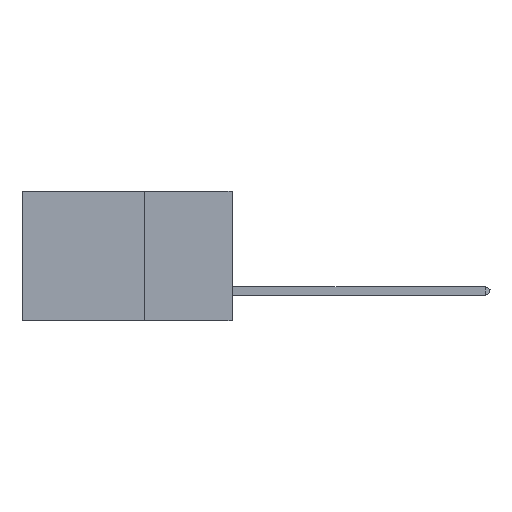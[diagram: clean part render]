
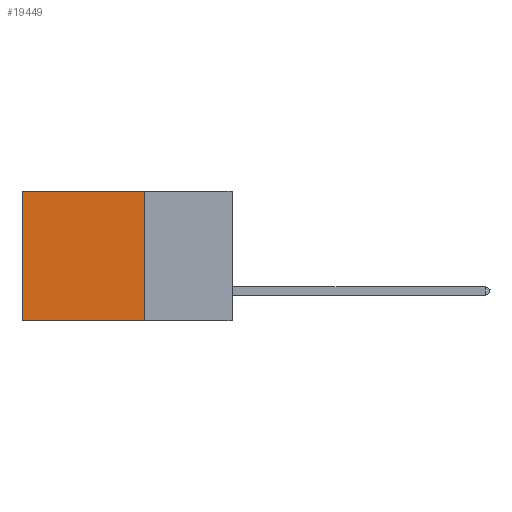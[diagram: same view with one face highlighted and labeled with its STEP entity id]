
A CAD part, left-side view. The second image highlights one B-rep face of the part: STEP entity #19449.
In plain terms, the highlighted planar face has unit normal (-1, 0, 0).
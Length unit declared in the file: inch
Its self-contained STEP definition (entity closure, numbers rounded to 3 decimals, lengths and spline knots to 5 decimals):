
#195 = ORIENTED_EDGE ( 'NONE', *, *, #9380, .F. ) ;
#300 = EDGE_CURVE ( 'NONE', #11918, #4703, #20986, .T. ) ;
#699 = VERTEX_POINT ( 'NONE', #17692 ) ;
#1132 = DIRECTION ( 'NONE',  ( 0., 1., 0. ) ) ;
#1620 = AXIS2_PLACEMENT_3D ( 'NONE', #14199, #4064, #3139 ) ;
#2274 = VERTEX_POINT ( 'NONE', #18508 ) ;
#2371 = EDGE_CURVE ( 'NONE', #4703, #2274, #4594, .T. ) ;
#3139 = DIRECTION ( 'NONE',  ( 0., 0., -1. ) ) ;
#3209 = CARTESIAN_POINT ( 'NONE',  ( 0.2875, 0.6, 0. ) ) ;
#3316 = CARTESIAN_POINT ( 'NONE',  ( 0.2875, 0.25, 0. ) ) ;
#3776 = CARTESIAN_POINT ( 'NONE',  ( 0.2875, 0.25, -0.37 ) ) ;
#4064 = DIRECTION ( 'NONE',  ( 1., 0., 0. ) ) ;
#4594 = LINE ( 'NONE', #5502, #14219 ) ;
#4656 = LINE ( 'NONE', #3316, #12672 ) ;
#4703 = VERTEX_POINT ( 'NONE', #3209 ) ;
#5502 = CARTESIAN_POINT ( 'NONE',  ( 0.2875, 0.6, 0. ) ) ;
#6002 = DIRECTION ( 'NONE',  ( 0., 1., 0. ) ) ;
#6985 = ORIENTED_EDGE ( 'NONE', *, *, #17021, .F. ) ;
#7794 = CARTESIAN_POINT ( 'NONE',  ( 0.2875, 0.25, 0. ) ) ;
#8422 = DIRECTION ( 'NONE',  ( 0., 0., -1. ) ) ;
#8754 = PLANE ( 'NONE',  #1620 ) ;
#9380 = EDGE_CURVE ( 'NONE', #699, #2274, #16230, .T. ) ;
#11918 = VERTEX_POINT ( 'NONE', #7794 ) ;
#12617 = FACE_OUTER_BOUND ( 'NONE', #18703, .T. ) ;
#12672 = VECTOR ( 'NONE', #8422, 39.37008 ) ;
#14199 = CARTESIAN_POINT ( 'NONE',  ( 0.2875, 0.25, 0. ) ) ;
#14219 = VECTOR ( 'NONE', #20794, 39.37008 ) ;
#16230 = LINE ( 'NONE', #3776, #19177 ) ;
#17021 = EDGE_CURVE ( 'NONE', #11918, #699, #4656, .T. ) ;
#17692 = CARTESIAN_POINT ( 'NONE',  ( 0.2875, 0.25, -0.37 ) ) ;
#18508 = CARTESIAN_POINT ( 'NONE',  ( 0.2875, 0.6, -0.37 ) ) ;
#18703 = EDGE_LOOP ( 'NONE', ( #20512, #195, #6985, #20201 ) ) ;
#19177 = VECTOR ( 'NONE', #1132, 39.37008 ) ;
#19416 = CARTESIAN_POINT ( 'NONE',  ( 0.2875, 0.25, 0. ) ) ;
#19449 = ADVANCED_FACE ( 'NONE', ( #12617 ), #8754, .F. ) ;
#19900 = VECTOR ( 'NONE', #6002, 39.37008 ) ;
#20201 = ORIENTED_EDGE ( 'NONE', *, *, #300, .T. ) ;
#20512 = ORIENTED_EDGE ( 'NONE', *, *, #2371, .T. ) ;
#20794 = DIRECTION ( 'NONE',  ( 0., 0., -1. ) ) ;
#20986 = LINE ( 'NONE', #19416, #19900 ) ;
